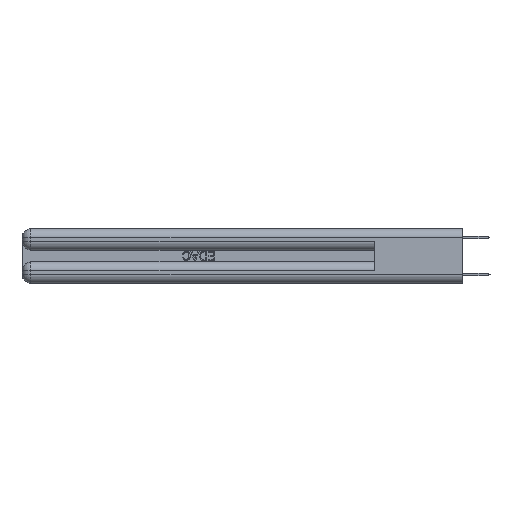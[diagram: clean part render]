
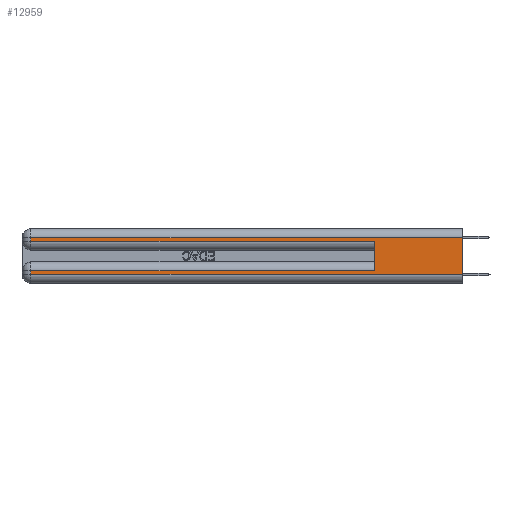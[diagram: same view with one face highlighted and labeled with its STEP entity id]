
A CAD part, left-side view. The second image highlights one B-rep face of the part: STEP entity #12959.
In plain terms, the highlighted planar face has unit normal (-1, 0, 0).
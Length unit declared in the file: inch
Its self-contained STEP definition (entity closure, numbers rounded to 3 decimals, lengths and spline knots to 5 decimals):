
#369 = DIRECTION ( 'NONE',  ( 0., 0., -1. ) ) ;
#596 = DIRECTION ( 'NONE',  ( 0., 1., 0. ) ) ;
#680 = LINE ( 'NONE', #28167, #26363 ) ;
#1294 = VERTEX_POINT ( 'NONE', #21523 ) ;
#1820 = VECTOR ( 'NONE', #26984, 39.37008 ) ;
#2075 = CARTESIAN_POINT ( 'NONE',  ( 0., 0., 0.06 ) ) ;
#2370 = DIRECTION ( 'NONE',  ( 0., 0., 1. ) ) ;
#2894 = CARTESIAN_POINT ( 'NONE',  ( 0., 0., 0.31 ) ) ;
#3076 = LINE ( 'NONE', #25210, #31888 ) ;
#3351 = DIRECTION ( 'NONE',  ( 0., -1., 0. ) ) ;
#3402 = ORIENTED_EDGE ( 'NONE', *, *, #8169, .T. ) ;
#3852 = VERTEX_POINT ( 'NONE', #7367 ) ;
#5350 = ORIENTED_EDGE ( 'NONE', *, *, #14434, .F. ) ;
#5793 = CARTESIAN_POINT ( 'NONE',  ( 0., 0.6, 0.285 ) ) ;
#7036 = CARTESIAN_POINT ( 'NONE',  ( 0., 2.94, 0.37 ) ) ;
#7367 = CARTESIAN_POINT ( 'NONE',  ( 0., 2.94, 0.31 ) ) ;
#7691 = VECTOR ( 'NONE', #596, 39.37008 ) ;
#7729 = CARTESIAN_POINT ( 'NONE',  ( 0., 2.94, 0.085 ) ) ;
#7978 = DIRECTION ( 'NONE',  ( 1., 0., 0. ) ) ;
#8036 = EDGE_CURVE ( 'NONE', #3852, #1294, #13232, .T. ) ;
#8169 = EDGE_CURVE ( 'NONE', #17072, #20564, #3076, .T. ) ;
#9700 = VERTEX_POINT ( 'NONE', #22055 ) ;
#11523 = EDGE_CURVE ( 'NONE', #9700, #15998, #21715, .T. ) ;
#11655 = LINE ( 'NONE', #18389, #27608 ) ;
#11753 = LINE ( 'NONE', #15235, #17646 ) ;
#12487 = CARTESIAN_POINT ( 'NONE',  ( 0., 0., 0.06 ) ) ;
#12959 = ADVANCED_FACE ( 'NONE', ( #30931 ), #18044, .F. ) ;
#13232 = LINE ( 'NONE', #7036, #24521 ) ;
#13628 = VERTEX_POINT ( 'NONE', #5793 ) ;
#14380 = ORIENTED_EDGE ( 'NONE', *, *, #8036, .T. ) ;
#14427 = VECTOR ( 'NONE', #31391, 39.37008 ) ;
#14434 = EDGE_CURVE ( 'NONE', #16968, #15998, #16436, .T. ) ;
#15235 = CARTESIAN_POINT ( 'NONE',  ( 0., 0.6, 0.145 ) ) ;
#15936 = EDGE_CURVE ( 'NONE', #17072, #13628, #11753, .T. ) ;
#15998 = VERTEX_POINT ( 'NONE', #12487 ) ;
#16436 = LINE ( 'NONE', #31186, #14427 ) ;
#16968 = VERTEX_POINT ( 'NONE', #20950 ) ;
#17072 = VERTEX_POINT ( 'NONE', #29174 ) ;
#17431 = AXIS2_PLACEMENT_3D ( 'NONE', #22927, #7978, #369 ) ;
#17646 = VECTOR ( 'NONE', #2370, 39.37008 ) ;
#18044 = PLANE ( 'NONE',  #17431 ) ;
#18389 = CARTESIAN_POINT ( 'NONE',  ( 0., 0., 0.285 ) ) ;
#18626 = LINE ( 'NONE', #2894, #7691 ) ;
#18926 = EDGE_LOOP ( 'NONE', ( #5350, #22075, #14380, #21008, #28724, #3402, #30261, #20371 ) ) ;
#19496 = DIRECTION ( 'NONE',  ( 0., 0., -1. ) ) ;
#20371 = ORIENTED_EDGE ( 'NONE', *, *, #11523, .T. ) ;
#20564 = VERTEX_POINT ( 'NONE', #7729 ) ;
#20950 = CARTESIAN_POINT ( 'NONE',  ( 0., 0., 0.31 ) ) ;
#21008 = ORIENTED_EDGE ( 'NONE', *, *, #23940, .T. ) ;
#21523 = CARTESIAN_POINT ( 'NONE',  ( 0., 2.94, 0.285 ) ) ;
#21715 = LINE ( 'NONE', #2075, #1820 ) ;
#22055 = CARTESIAN_POINT ( 'NONE',  ( 0., 2.94, 0.06 ) ) ;
#22075 = ORIENTED_EDGE ( 'NONE', *, *, #25006, .T. ) ;
#22927 = CARTESIAN_POINT ( 'NONE',  ( 0., 0., 0.37 ) ) ;
#22985 = DIRECTION ( 'NONE',  ( 0., 0., -1. ) ) ;
#23940 = EDGE_CURVE ( 'NONE', #1294, #13628, #11655, .T. ) ;
#24521 = VECTOR ( 'NONE', #19496, 39.37008 ) ;
#25006 = EDGE_CURVE ( 'NONE', #16968, #3852, #18626, .T. ) ;
#25210 = CARTESIAN_POINT ( 'NONE',  ( 0., 0., 0.085 ) ) ;
#26363 = VECTOR ( 'NONE', #22985, 39.37008 ) ;
#26984 = DIRECTION ( 'NONE',  ( 0., -1., 0. ) ) ;
#27608 = VECTOR ( 'NONE', #3351, 39.37008 ) ;
#28167 = CARTESIAN_POINT ( 'NONE',  ( 0., 2.94, 0.37 ) ) ;
#28724 = ORIENTED_EDGE ( 'NONE', *, *, #15936, .F. ) ;
#29174 = CARTESIAN_POINT ( 'NONE',  ( 0., 0.6, 0.085 ) ) ;
#29978 = EDGE_CURVE ( 'NONE', #20564, #9700, #680, .T. ) ;
#30115 = DIRECTION ( 'NONE',  ( 0., 1., 0. ) ) ;
#30261 = ORIENTED_EDGE ( 'NONE', *, *, #29978, .T. ) ;
#30931 = FACE_OUTER_BOUND ( 'NONE', #18926, .T. ) ;
#31186 = CARTESIAN_POINT ( 'NONE',  ( 0., 0., 0.37 ) ) ;
#31391 = DIRECTION ( 'NONE',  ( 0., 0., -1. ) ) ;
#31888 = VECTOR ( 'NONE', #30115, 39.37008 ) ;
